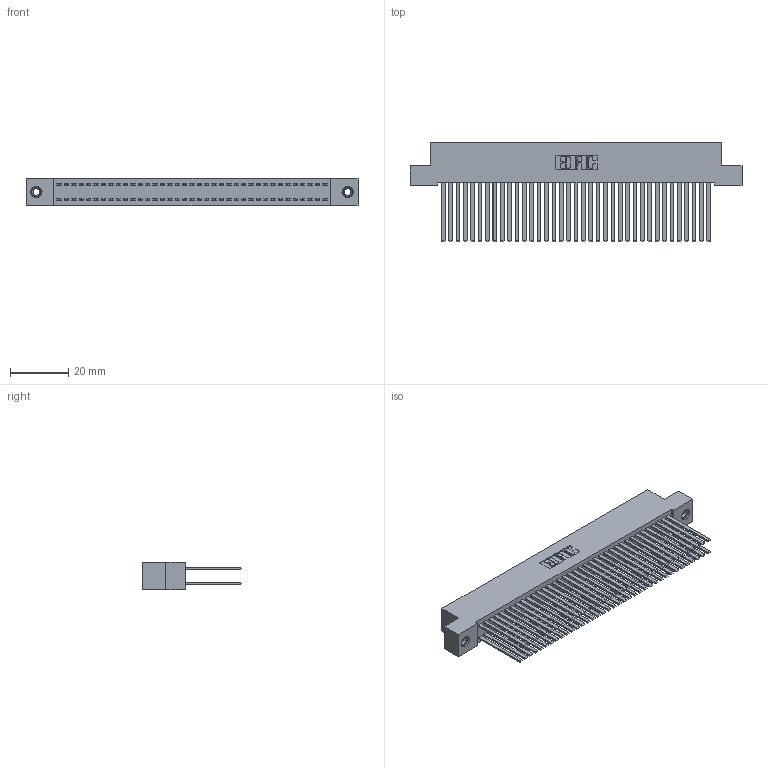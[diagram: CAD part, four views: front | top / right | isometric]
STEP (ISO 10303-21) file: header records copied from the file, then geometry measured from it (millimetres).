
FILE_DESCRIPTION (( 'STEP AP203' ), '1' );
FILE_NAME ('392-074-544-208.STEP', '2019-10-09T13:06:36', ( '' ), ( '' ), 'SwSTEP 2.0', 'SolidWorks 2016', '' );
FILE_SCHEMA (( 'CONFIG_CONTROL_DESIGN' ));
Length unit declared in the file: inch
Products named in the file (4): 342 Part_TI; 345-292-001_345-293-144; 345-250-001_345-250-003-102; 392-074-544-208
Assembly tree (77 placements, depth 2):
  392-074-544-208
    342 Part_TI
    345-292-001_345-293-144  x74
    345-250-001_345-250-003-102  x2
Bounding box: 114.3 x 34.3 x 9.4 mm (x, y, z)
Volume: 11277.8 mm3; surface area: 21117.3 mm2
Topology: 77 solids, 77 shells, 3574 faces, 10573 edges, 6942 vertices
Faces by surface type: plane 2466, cylinder 1092, cone 12, torus 4
Entity records: 25320 total; most frequent: CARTESIAN_POINT 4181, ORIENTED_EDGE 4110, DIRECTION 3609, EDGE_CURVE 2055, LINE 1911, VECTOR 1911, VERTEX_POINT 1364, AXIS2_PLACEMENT_3D 849
